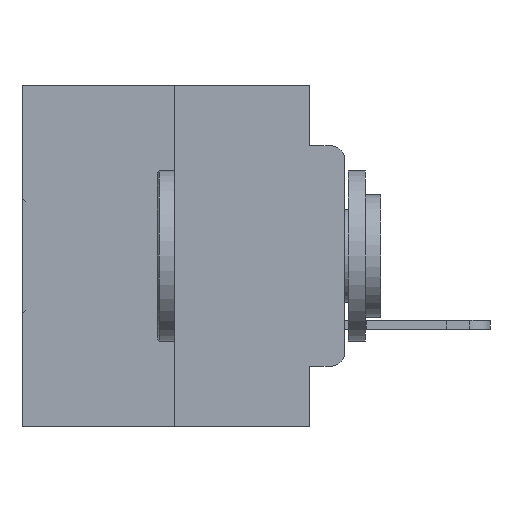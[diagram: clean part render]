
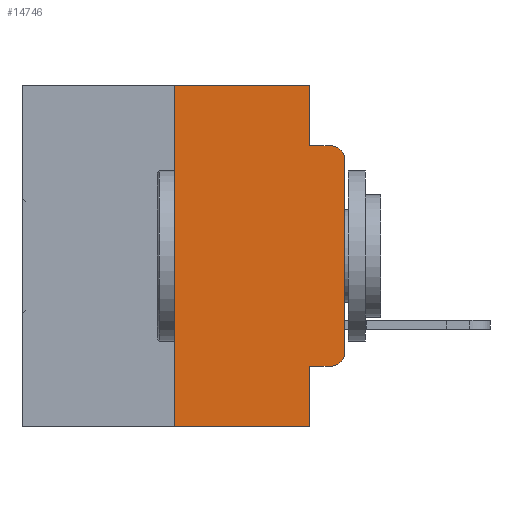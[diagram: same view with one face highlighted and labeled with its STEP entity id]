
A CAD part, left-side view. The second image highlights one B-rep face of the part: STEP entity #14746.
In plain terms, the highlighted planar face has unit normal (-1, 0, 0).
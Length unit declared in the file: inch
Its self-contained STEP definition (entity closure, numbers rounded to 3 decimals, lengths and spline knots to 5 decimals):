
#372 = CARTESIAN_POINT ( 'NONE',  ( 0., 0., -0.1085 ) ) ;
#690 = LINE ( 'NONE', #22077, #7270 ) ;
#1536 = VECTOR ( 'NONE', #6353, 39.37008 ) ;
#1883 = DIRECTION ( 'NONE',  ( 0., -1., 0. ) ) ;
#2081 = AXIS2_PLACEMENT_3D ( 'NONE', #22271, #22164, #22066 ) ;
#2303 = VERTEX_POINT ( 'NONE', #4117 ) ;
#2441 = CARTESIAN_POINT ( 'NONE',  ( 0., 0.051, -0.0885 ) ) ;
#2446 = LINE ( 'NONE', #6605, #1536 ) ;
#3139 = CARTESIAN_POINT ( 'NONE',  ( 0., 0.25, 0. ) ) ;
#3400 = LINE ( 'NONE', #2441, #4243 ) ;
#3446 = VERTEX_POINT ( 'NONE', #27732 ) ;
#3828 = LINE ( 'NONE', #3139, #29900 ) ;
#4117 = CARTESIAN_POINT ( 'NONE',  ( 0., 0.02, -0.4115 ) ) ;
#4243 = VECTOR ( 'NONE', #1883, 39.37008 ) ;
#4465 = VERTEX_POINT ( 'NONE', #7945 ) ;
#4553 = CARTESIAN_POINT ( 'NONE',  ( 0., 0.051, 0. ) ) ;
#4561 = ORIENTED_EDGE ( 'NONE', *, *, #22659, .T. ) ;
#4639 = EDGE_CURVE ( 'NONE', #28734, #30435, #3400, .T. ) ;
#4781 = ORIENTED_EDGE ( 'NONE', *, *, #8640, .F. ) ;
#4853 = VECTOR ( 'NONE', #13946, 39.37008 ) ;
#6353 = DIRECTION ( 'NONE',  ( 0., -1., 0. ) ) ;
#6385 = ORIENTED_EDGE ( 'NONE', *, *, #31909, .F. ) ;
#6536 = EDGE_CURVE ( 'NONE', #19934, #30435, #22778, .T. ) ;
#6557 = ORIENTED_EDGE ( 'NONE', *, *, #30519, .F. ) ;
#6605 = CARTESIAN_POINT ( 'NONE',  ( 0., 0.473, -0.5 ) ) ;
#7270 = VECTOR ( 'NONE', #19595, 39.37008 ) ;
#7371 = ORIENTED_EDGE ( 'NONE', *, *, #14002, .T. ) ;
#7945 = CARTESIAN_POINT ( 'NONE',  ( 0., 0.25, 0. ) ) ;
#8153 = ORIENTED_EDGE ( 'NONE', *, *, #24379, .F. ) ;
#8640 = EDGE_CURVE ( 'NONE', #4465, #24815, #23420, .T. ) ;
#8780 = CARTESIAN_POINT ( 'NONE',  ( 0., 0.051, -0.4115 ) ) ;
#9379 = DIRECTION ( 'NONE',  ( 0., 0., -1. ) ) ;
#9568 = DIRECTION ( 'NONE',  ( -1., 0., 0. ) ) ;
#9839 = AXIS2_PLACEMENT_3D ( 'NONE', #10009, #9568, #9379 ) ;
#10009 = CARTESIAN_POINT ( 'NONE',  ( 0., 0.02, -0.1085 ) ) ;
#10073 = EDGE_CURVE ( 'NONE', #3446, #19934, #17449, .T. ) ;
#12311 = DIRECTION ( 'NONE',  ( 0., 0., -1. ) ) ;
#12499 = CARTESIAN_POINT ( 'NONE',  ( 0., 0.02, -0.3915 ) ) ;
#12953 = AXIS2_PLACEMENT_3D ( 'NONE', #12499, #13406, #12311 ) ;
#13406 = DIRECTION ( 'NONE',  ( -1., 0., 0. ) ) ;
#13532 = VECTOR ( 'NONE', #27611, 39.37008 ) ;
#13946 = DIRECTION ( 'NONE',  ( 0., -1., 0. ) ) ;
#14002 = EDGE_CURVE ( 'NONE', #23034, #30574, #2446, .T. ) ;
#14746 = ADVANCED_FACE ( 'NONE', ( #18830 ), #23247, .F. ) ;
#15084 = ORIENTED_EDGE ( 'NONE', *, *, #4639, .F. ) ;
#16089 = CARTESIAN_POINT ( 'NONE',  ( 0., 0.02, -0.0885 ) ) ;
#16791 = CARTESIAN_POINT ( 'NONE',  ( 0., 0.473, 0. ) ) ;
#17184 = DIRECTION ( 'NONE',  ( 0., -1., 0. ) ) ;
#17449 = LINE ( 'NONE', #32366, #30256 ) ;
#18252 = CARTESIAN_POINT ( 'NONE',  ( 0., 0.051, -0.0885 ) ) ;
#18830 = FACE_OUTER_BOUND ( 'NONE', #29499, .T. ) ;
#19595 = DIRECTION ( 'NONE',  ( 0., 0., -1. ) ) ;
#19934 = VERTEX_POINT ( 'NONE', #372 ) ;
#20164 = CARTESIAN_POINT ( 'NONE',  ( 0., 0.051, -0.4115 ) ) ;
#20320 = LINE ( 'NONE', #4553, #13532 ) ;
#21015 = EDGE_CURVE ( 'NONE', #2303, #3446, #23619, .T. ) ;
#21501 = CARTESIAN_POINT ( 'NONE',  ( 0., 0.051, -0.5 ) ) ;
#21814 = VERTEX_POINT ( 'NONE', #20164 ) ;
#22066 = DIRECTION ( 'NONE',  ( 0., 0., -1. ) ) ;
#22077 = CARTESIAN_POINT ( 'NONE',  ( 0., 0.051, 0. ) ) ;
#22164 = DIRECTION ( 'NONE',  ( 1., 0., 0. ) ) ;
#22271 = CARTESIAN_POINT ( 'NONE',  ( 0., 0.473, 0. ) ) ;
#22608 = VECTOR ( 'NONE', #17184, 39.37008 ) ;
#22651 = CARTESIAN_POINT ( 'NONE',  ( 0., 0.25, -0.5 ) ) ;
#22659 = EDGE_CURVE ( 'NONE', #21814, #2303, #31389, .T. ) ;
#22778 = CIRCLE ( 'NONE', #9839, 0.02 ) ;
#23034 = VERTEX_POINT ( 'NONE', #22651 ) ;
#23247 = PLANE ( 'NONE',  #2081 ) ;
#23419 = ORIENTED_EDGE ( 'NONE', *, *, #10073, .T. ) ;
#23420 = LINE ( 'NONE', #16791, #22608 ) ;
#23619 = CIRCLE ( 'NONE', #12953, 0.02 ) ;
#23969 = ORIENTED_EDGE ( 'NONE', *, *, #6536, .T. ) ;
#24379 = EDGE_CURVE ( 'NONE', #21814, #30574, #20320, .T. ) ;
#24815 = VERTEX_POINT ( 'NONE', #27001 ) ;
#26355 = DIRECTION ( 'NONE',  ( 0., 0., 1. ) ) ;
#27001 = CARTESIAN_POINT ( 'NONE',  ( 0., 0.051, 0. ) ) ;
#27611 = DIRECTION ( 'NONE',  ( 0., 0., -1. ) ) ;
#27732 = CARTESIAN_POINT ( 'NONE',  ( 0., 0., -0.3915 ) ) ;
#27947 = ORIENTED_EDGE ( 'NONE', *, *, #21015, .T. ) ;
#28734 = VERTEX_POINT ( 'NONE', #18252 ) ;
#29499 = EDGE_LOOP ( 'NONE', ( #23419, #23969, #15084, #6385, #4781, #6557, #7371, #8153, #4561, #27947 ) ) ;
#29900 = VECTOR ( 'NONE', #26355, 39.37008 ) ;
#30256 = VECTOR ( 'NONE', #31061, 39.37008 ) ;
#30435 = VERTEX_POINT ( 'NONE', #16089 ) ;
#30519 = EDGE_CURVE ( 'NONE', #23034, #4465, #3828, .T. ) ;
#30574 = VERTEX_POINT ( 'NONE', #21501 ) ;
#31061 = DIRECTION ( 'NONE',  ( 0., 0., 1. ) ) ;
#31389 = LINE ( 'NONE', #8780, #4853 ) ;
#31909 = EDGE_CURVE ( 'NONE', #24815, #28734, #690, .T. ) ;
#32366 = CARTESIAN_POINT ( 'NONE',  ( 0., 0., 0. ) ) ;
